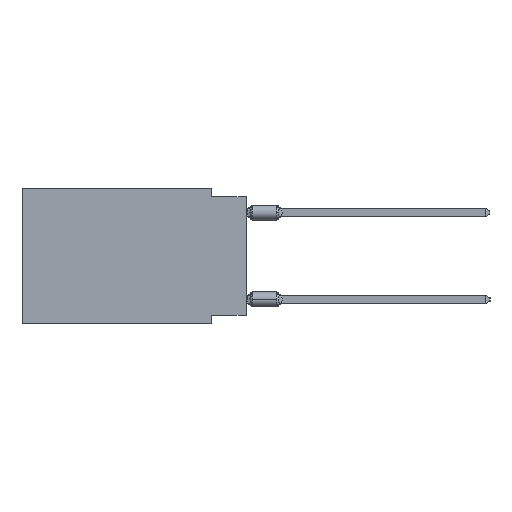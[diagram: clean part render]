
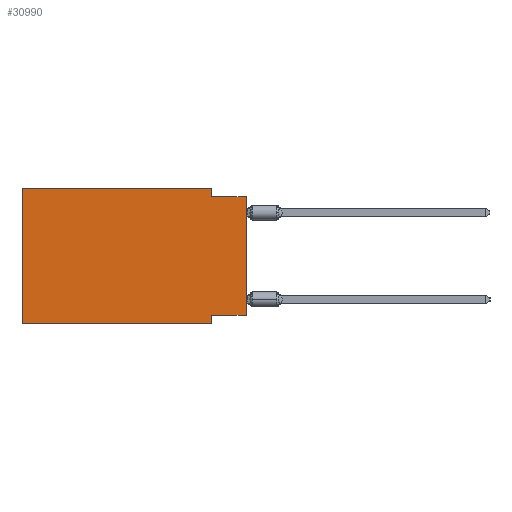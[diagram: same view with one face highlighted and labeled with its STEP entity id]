
A CAD part, left-side view. The second image highlights one B-rep face of the part: STEP entity #30990.
In plain terms, the highlighted planar face has unit normal (-1, 0, 0).
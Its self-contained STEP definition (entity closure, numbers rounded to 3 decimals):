
#812 = CARTESIAN_POINT ( 'NONE',  ( 0., 16.383, 0. ) ) ;
#2000 = LINE ( 'NONE', #40814, #60217 ) ;
#2014 = VECTOR ( 'NONE', #10728, 1000. ) ;
#2394 = CARTESIAN_POINT ( 'NONE',  ( 0., 0., -9.271 ) ) ;
#3149 = ORIENTED_EDGE ( 'NONE', *, *, #5962, .F. ) ;
#3428 = VERTEX_POINT ( 'NONE', #2394 ) ;
#4227 = VECTOR ( 'NONE', #34933, 1000. ) ;
#5962 = EDGE_CURVE ( 'NONE', #29279, #32861, #51254, .T. ) ;
#7305 = CARTESIAN_POINT ( 'NONE',  ( 0., 0., -0.635 ) ) ;
#8125 = ORIENTED_EDGE ( 'NONE', *, *, #25480, .T. ) ;
#9615 = CARTESIAN_POINT ( 'NONE',  ( 0., 2.54, -9.906 ) ) ;
#9909 = CARTESIAN_POINT ( 'NONE',  ( 0., 16.383, -9.906 ) ) ;
#10728 = DIRECTION ( 'NONE',  ( 0., 0., -1. ) ) ;
#11422 = ORIENTED_EDGE ( 'NONE', *, *, #12123, .F. ) ;
#12123 = EDGE_CURVE ( 'NONE', #37155, #33450, #59519, .T. ) ;
#13974 = EDGE_CURVE ( 'NONE', #3428, #47156, #2000, .T. ) ;
#15786 = FACE_OUTER_BOUND ( 'NONE', #52294, .T. ) ;
#17645 = VECTOR ( 'NONE', #34965, 1000. ) ;
#18784 = ORIENTED_EDGE ( 'NONE', *, *, #25818, .F. ) ;
#19111 = DIRECTION ( 'NONE',  ( 0., -1., 0. ) ) ;
#20481 = VECTOR ( 'NONE', #42187, 1000. ) ;
#22301 = CARTESIAN_POINT ( 'NONE',  ( 0., 0., 0. ) ) ;
#23807 = AXIS2_PLACEMENT_3D ( 'NONE', #54916, #54288, #39522 ) ;
#24244 = LINE ( 'NONE', #24564, #38623 ) ;
#24564 = CARTESIAN_POINT ( 'NONE',  ( 0., 16.383, 0. ) ) ;
#25480 = EDGE_CURVE ( 'NONE', #3428, #32861, #51179, .T. ) ;
#25818 = EDGE_CURVE ( 'NONE', #45261, #29279, #59492, .T. ) ;
#26865 = DIRECTION ( 'NONE',  ( 0., -1., 0. ) ) ;
#27319 = EDGE_CURVE ( 'NONE', #47156, #28947, #43917, .T. ) ;
#28947 = VERTEX_POINT ( 'NONE', #9615 ) ;
#29279 = VERTEX_POINT ( 'NONE', #53425 ) ;
#29800 = CARTESIAN_POINT ( 'NONE',  ( 0., 2.54, -9.906 ) ) ;
#30771 = CARTESIAN_POINT ( 'NONE',  ( 0., 16.383, -9.906 ) ) ;
#30990 = ADVANCED_FACE ( 'NONE', ( #15786 ), #40775, .F. ) ;
#32861 = VERTEX_POINT ( 'NONE', #58330 ) ;
#33450 = VERTEX_POINT ( 'NONE', #50123 ) ;
#33557 = VECTOR ( 'NONE', #26865, 1000. ) ;
#34189 = DIRECTION ( 'NONE',  ( 0., 0., 1. ) ) ;
#34414 = EDGE_CURVE ( 'NONE', #33450, #45261, #24244, .T. ) ;
#34933 = DIRECTION ( 'NONE',  ( 0., 0., -1. ) ) ;
#34965 = DIRECTION ( 'NONE',  ( 0., -1., 0. ) ) ;
#35293 = ORIENTED_EDGE ( 'NONE', *, *, #39044, .T. ) ;
#37155 = VERTEX_POINT ( 'NONE', #9909 ) ;
#38623 = VECTOR ( 'NONE', #19111, 1000. ) ;
#39044 = EDGE_CURVE ( 'NONE', #37155, #28947, #49088, .T. ) ;
#39522 = DIRECTION ( 'NONE',  ( 0., 0., -1. ) ) ;
#39679 = ORIENTED_EDGE ( 'NONE', *, *, #34414, .F. ) ;
#40535 = CARTESIAN_POINT ( 'NONE',  ( 0., 2.54, 0. ) ) ;
#40775 = PLANE ( 'NONE',  #23807 ) ;
#40814 = CARTESIAN_POINT ( 'NONE',  ( 0., 0., -9.271 ) ) ;
#41859 = ORIENTED_EDGE ( 'NONE', *, *, #27319, .F. ) ;
#42187 = DIRECTION ( 'NONE',  ( 0., 0., 1. ) ) ;
#43917 = LINE ( 'NONE', #29800, #4227 ) ;
#45261 = VERTEX_POINT ( 'NONE', #56044 ) ;
#45448 = ORIENTED_EDGE ( 'NONE', *, *, #13974, .F. ) ;
#45737 = VECTOR ( 'NONE', #34189, 1000. ) ;
#47156 = VERTEX_POINT ( 'NONE', #51354 ) ;
#49088 = LINE ( 'NONE', #30771, #17645 ) ;
#50123 = CARTESIAN_POINT ( 'NONE',  ( 0., 16.383, 0. ) ) ;
#50440 = DIRECTION ( 'NONE',  ( 0., 1., 0. ) ) ;
#51179 = LINE ( 'NONE', #22301, #20481 ) ;
#51254 = LINE ( 'NONE', #7305, #33557 ) ;
#51354 = CARTESIAN_POINT ( 'NONE',  ( 0., 2.54, -9.271 ) ) ;
#52294 = EDGE_LOOP ( 'NONE', ( #8125, #3149, #18784, #39679, #11422, #35293, #41859, #45448 ) ) ;
#53425 = CARTESIAN_POINT ( 'NONE',  ( 0., 2.54, -0.635 ) ) ;
#54288 = DIRECTION ( 'NONE',  ( 1., 0., 0. ) ) ;
#54916 = CARTESIAN_POINT ( 'NONE',  ( 0., 16.383, 0. ) ) ;
#56044 = CARTESIAN_POINT ( 'NONE',  ( 0., 2.54, 0. ) ) ;
#58330 = CARTESIAN_POINT ( 'NONE',  ( 0., 0., -0.635 ) ) ;
#59492 = LINE ( 'NONE', #40535, #2014 ) ;
#59519 = LINE ( 'NONE', #812, #45737 ) ;
#60217 = VECTOR ( 'NONE', #50440, 1000. ) ;
